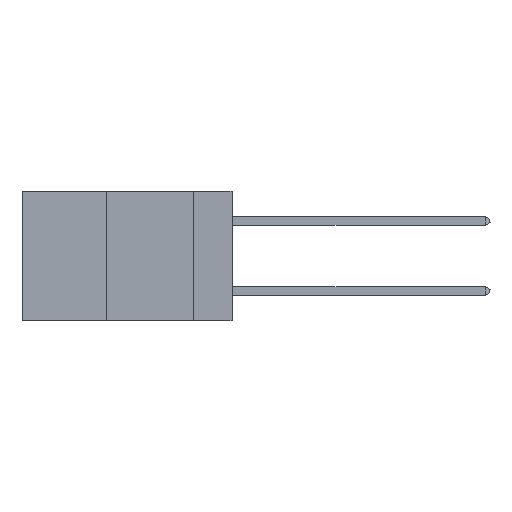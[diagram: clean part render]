
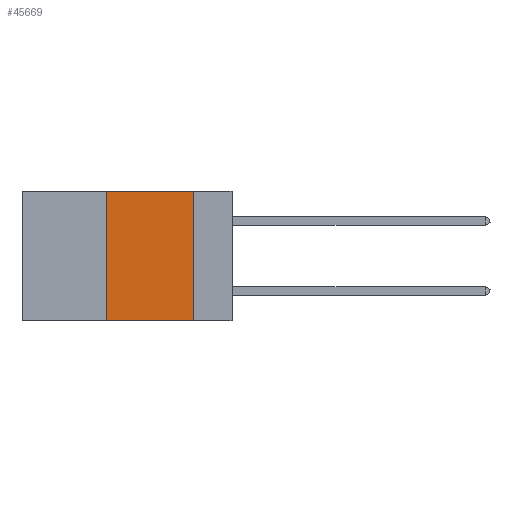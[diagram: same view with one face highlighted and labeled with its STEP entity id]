
A CAD part, left-side view. The second image highlights one B-rep face of the part: STEP entity #45669.
In plain terms, the highlighted planar face has unit normal (-1, 0, 0).
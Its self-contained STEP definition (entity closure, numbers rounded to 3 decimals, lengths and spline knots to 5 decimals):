
#48 = PLANE ( 'NONE',  #46110 ) ;
#301 = LINE ( 'NONE', #28707, #3646 ) ;
#2307 = VECTOR ( 'NONE', #24772, 39.37008 ) ;
#3646 = VECTOR ( 'NONE', #11003, 39.37008 ) ;
#6368 = CARTESIAN_POINT ( 'NONE',  ( 0., 0.11, -0.37 ) ) ;
#11003 = DIRECTION ( 'NONE',  ( 0., -1., 0. ) ) ;
#13540 = DIRECTION ( 'NONE',  ( 0., 0., 1. ) ) ;
#14317 = VECTOR ( 'NONE', #13540, 39.37008 ) ;
#14829 = ORIENTED_EDGE ( 'NONE', *, *, #15057, .F. ) ;
#15057 = EDGE_CURVE ( 'NONE', #36054, #23832, #37782, .T. ) ;
#16676 = LINE ( 'NONE', #19372, #29694 ) ;
#18200 = ORIENTED_EDGE ( 'NONE', *, *, #26393, .T. ) ;
#19372 = CARTESIAN_POINT ( 'NONE',  ( 0., 0.6, -0.37 ) ) ;
#21421 = CARTESIAN_POINT ( 'NONE',  ( 0., 0.6, 0. ) ) ;
#23044 = EDGE_CURVE ( 'NONE', #46159, #36054, #301, .T. ) ;
#23151 = DIRECTION ( 'NONE',  ( 0., -1., 0. ) ) ;
#23617 = CARTESIAN_POINT ( 'NONE',  ( 0., 0.36, 0. ) ) ;
#23832 = VERTEX_POINT ( 'NONE', #6368 ) ;
#24772 = DIRECTION ( 'NONE',  ( 0., 0., -1. ) ) ;
#24951 = CARTESIAN_POINT ( 'NONE',  ( 0., 0.11, 0. ) ) ;
#26393 = EDGE_CURVE ( 'NONE', #39864, #23832, #16676, .T. ) ;
#26709 = CARTESIAN_POINT ( 'NONE',  ( 0., 0.36, -0.37 ) ) ;
#27227 = EDGE_CURVE ( 'NONE', #39864, #46159, #32363, .T. ) ;
#28131 = ORIENTED_EDGE ( 'NONE', *, *, #27227, .F. ) ;
#28405 = CARTESIAN_POINT ( 'NONE',  ( 0., 0.11, 0. ) ) ;
#28707 = CARTESIAN_POINT ( 'NONE',  ( 0., 0.6, 0. ) ) ;
#29694 = VECTOR ( 'NONE', #23151, 39.37008 ) ;
#31833 = CARTESIAN_POINT ( 'NONE',  ( 0., 0.36, 0. ) ) ;
#31835 = DIRECTION ( 'NONE',  ( 0., 0., -1. ) ) ;
#32363 = LINE ( 'NONE', #31833, #14317 ) ;
#32866 = EDGE_LOOP ( 'NONE', ( #14829, #39694, #28131, #18200 ) ) ;
#35882 = DIRECTION ( 'NONE',  ( 1., 0., 0. ) ) ;
#36054 = VERTEX_POINT ( 'NONE', #24951 ) ;
#37782 = LINE ( 'NONE', #28405, #2307 ) ;
#38290 = FACE_OUTER_BOUND ( 'NONE', #32866, .T. ) ;
#39694 = ORIENTED_EDGE ( 'NONE', *, *, #23044, .F. ) ;
#39864 = VERTEX_POINT ( 'NONE', #26709 ) ;
#45669 = ADVANCED_FACE ( 'NONE', ( #38290 ), #48, .F. ) ;
#46110 = AXIS2_PLACEMENT_3D ( 'NONE', #21421, #35882, #31835 ) ;
#46159 = VERTEX_POINT ( 'NONE', #23617 ) ;
